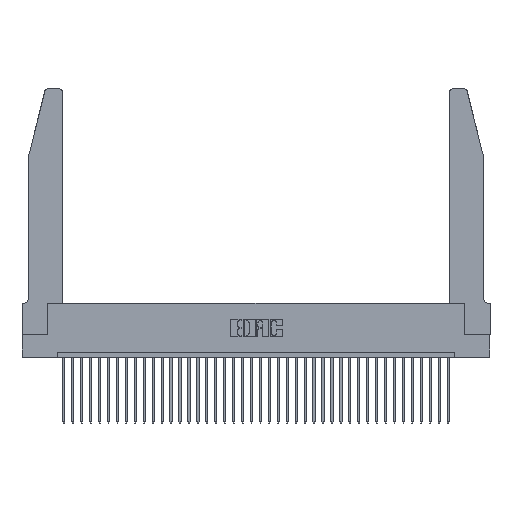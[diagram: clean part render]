
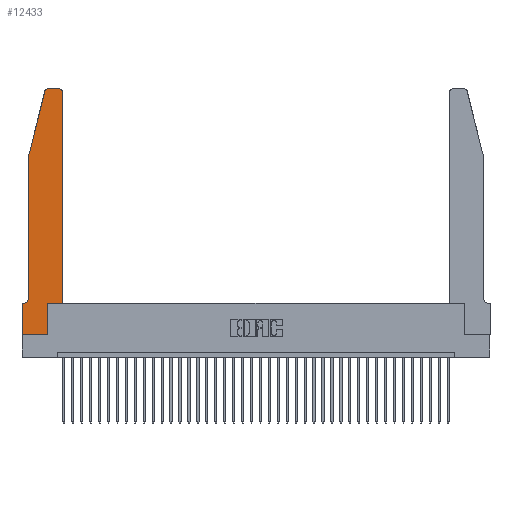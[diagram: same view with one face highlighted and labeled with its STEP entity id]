
A CAD part, top view. The second image highlights one B-rep face of the part: STEP entity #12433.
In plain terms, the highlighted planar face has unit normal (0, 0, 1).
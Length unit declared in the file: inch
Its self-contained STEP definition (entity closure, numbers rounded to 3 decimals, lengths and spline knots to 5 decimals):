
#26 = DIRECTION ( 'NONE',  ( -1., 0., 0. ) ) ;
#142 = DIRECTION ( 'NONE',  ( 0., 0., -1. ) ) ;
#622 = VERTEX_POINT ( 'NONE', #20012 ) ;
#1090 = CARTESIAN_POINT ( 'NONE',  ( 0.0755, 2., 0.37 ) ) ;
#2080 = EDGE_CURVE ( 'NONE', #25891, #23656, #34438, .T. ) ;
#2260 = CARTESIAN_POINT ( 'NONE',  ( 0.2865, 0.35, 0.37 ) ) ;
#3184 = ORIENTED_EDGE ( 'NONE', *, *, #5384, .T. ) ;
#3416 = VECTOR ( 'NONE', #31844, 39.37008 ) ;
#3446 = CARTESIAN_POINT ( 'NONE',  ( 0.4505, 2.72, 0.37 ) ) ;
#4374 = DIRECTION ( 'NONE',  ( 1., 0., 0. ) ) ;
#4702 = PLANE ( 'NONE',  #23932 ) ;
#4921 = VECTOR ( 'NONE', #36363, 39.37008 ) ;
#5002 = LINE ( 'NONE', #12456, #34992 ) ;
#5061 = ORIENTED_EDGE ( 'NONE', *, *, #16618, .T. ) ;
#5384 = EDGE_CURVE ( 'NONE', #24776, #35681, #33946, .T. ) ;
#5389 = VERTEX_POINT ( 'NONE', #29355 ) ;
#5837 = EDGE_CURVE ( 'NONE', #5389, #24776, #26176, .T. ) ;
#6209 = AXIS2_PLACEMENT_3D ( 'NONE', #10601, #16093, #4374 ) ;
#7248 = ORIENTED_EDGE ( 'NONE', *, *, #21227, .T. ) ;
#7262 = VECTOR ( 'NONE', #21818, 39.37008 ) ;
#7862 = CARTESIAN_POINT ( 'NONE',  ( 0.0055, 0.42, 0.37 ) ) ;
#8034 = CARTESIAN_POINT ( 'NONE',  ( 0., 0., 0.37 ) ) ;
#8630 = CIRCLE ( 'NONE', #18538, 0.07 ) ;
#8781 = CARTESIAN_POINT ( 'NONE',  ( 0.0055, 0.35, 0.37 ) ) ;
#8785 = EDGE_LOOP ( 'NONE', ( #16765, #20281, #16480, #3184, #7248, #9335, #5061, #36417, #18719, #33407, #26424, #9458 ) ) ;
#9014 = DIRECTION ( 'NONE',  ( 0., -1., 0. ) ) ;
#9170 = EDGE_CURVE ( 'NONE', #14388, #25891, #5002, .T. ) ;
#9207 = LINE ( 'NONE', #15293, #27850 ) ;
#9335 = ORIENTED_EDGE ( 'NONE', *, *, #14535, .T. ) ;
#9458 = ORIENTED_EDGE ( 'NONE', *, *, #36519, .T. ) ;
#10260 = CARTESIAN_POINT ( 'NONE',  ( 0., 0., 0.37 ) ) ;
#10601 = CARTESIAN_POINT ( 'NONE',  ( 0.284, 2.72, 0.37 ) ) ;
#10736 = CARTESIAN_POINT ( 'NONE',  ( 0.4505, 0.35, 0.37 ) ) ;
#11313 = EDGE_CURVE ( 'NONE', #13683, #11473, #19161, .T. ) ;
#11473 = VERTEX_POINT ( 'NONE', #37413 ) ;
#11820 = DIRECTION ( 'NONE',  ( 0., 0., 1. ) ) ;
#12433 = ADVANCED_FACE ( 'NONE', ( #17025 ), #4702, .T. ) ;
#12456 = CARTESIAN_POINT ( 'NONE',  ( 0.4505, 0.35, 0.37 ) ) ;
#12545 = EDGE_CURVE ( 'NONE', #25888, #22016, #34281, .T. ) ;
#13468 = DIRECTION ( 'NONE',  ( 0., 0., 1. ) ) ;
#13683 = VERTEX_POINT ( 'NONE', #8034 ) ;
#13939 = CIRCLE ( 'NONE', #15026, 0.03 ) ;
#14279 = VERTEX_POINT ( 'NONE', #8781 ) ;
#14388 = VERTEX_POINT ( 'NONE', #2260 ) ;
#14535 = EDGE_CURVE ( 'NONE', #14279, #622, #29141, .T. ) ;
#15026 = AXIS2_PLACEMENT_3D ( 'NONE', #23036, #11820, #17715 ) ;
#15293 = CARTESIAN_POINT ( 'NONE',  ( 0.2865, 0.35, 0.37 ) ) ;
#15770 = VECTOR ( 'NONE', #9014, 39.37008 ) ;
#16093 = DIRECTION ( 'NONE',  ( 0., 0., 1. ) ) ;
#16480 = ORIENTED_EDGE ( 'NONE', *, *, #5837, .T. ) ;
#16618 = EDGE_CURVE ( 'NONE', #622, #13683, #26628, .T. ) ;
#16765 = ORIENTED_EDGE ( 'NONE', *, *, #12545, .T. ) ;
#17025 = FACE_OUTER_BOUND ( 'NONE', #8785, .T. ) ;
#17715 = DIRECTION ( 'NONE',  ( 1., 0., 0. ) ) ;
#18538 = AXIS2_PLACEMENT_3D ( 'NONE', #7862, #142, #26 ) ;
#18719 = ORIENTED_EDGE ( 'NONE', *, *, #26531, .T. ) ;
#18744 = CARTESIAN_POINT ( 'NONE',  ( 0.4505, 0.35, 0.37 ) ) ;
#19161 = LINE ( 'NONE', #25100, #7262 ) ;
#19761 = CARTESIAN_POINT ( 'NONE',  ( 0.4205, 2.75, 0.37 ) ) ;
#20012 = CARTESIAN_POINT ( 'NONE',  ( 0., 0.35, 0.37 ) ) ;
#20281 = ORIENTED_EDGE ( 'NONE', *, *, #36299, .T. ) ;
#20335 = CARTESIAN_POINT ( 'NONE',  ( 0.0755, 0.35, 0.37 ) ) ;
#21227 = EDGE_CURVE ( 'NONE', #35681, #14279, #8630, .T. ) ;
#21818 = DIRECTION ( 'NONE',  ( 1., 0., 0. ) ) ;
#21905 = DIRECTION ( 'NONE',  ( 1., 0., 0. ) ) ;
#22016 = VERTEX_POINT ( 'NONE', #23420 ) ;
#23036 = CARTESIAN_POINT ( 'NONE',  ( 0.4205, 2.72, 0.37 ) ) ;
#23420 = CARTESIAN_POINT ( 'NONE',  ( 0.284, 2.75, 0.37 ) ) ;
#23656 = VERTEX_POINT ( 'NONE', #3446 ) ;
#23932 = AXIS2_PLACEMENT_3D ( 'NONE', #30872, #13468, #21905 ) ;
#24088 = CIRCLE ( 'NONE', #6209, 0.03 ) ;
#24591 = VECTOR ( 'NONE', #34892, 39.37008 ) ;
#24765 = VECTOR ( 'NONE', #37328, 39.37008 ) ;
#24776 = VERTEX_POINT ( 'NONE', #1090 ) ;
#25100 = CARTESIAN_POINT ( 'NONE',  ( 0., 0., 0.37 ) ) ;
#25888 = VERTEX_POINT ( 'NONE', #19761 ) ;
#25891 = VERTEX_POINT ( 'NONE', #10736 ) ;
#26176 = LINE ( 'NONE', #32086, #3416 ) ;
#26207 = VECTOR ( 'NONE', #30218, 39.37008 ) ;
#26424 = ORIENTED_EDGE ( 'NONE', *, *, #2080, .T. ) ;
#26531 = EDGE_CURVE ( 'NONE', #11473, #14388, #9207, .T. ) ;
#26628 = LINE ( 'NONE', #10260, #26207 ) ;
#27850 = VECTOR ( 'NONE', #35589, 39.37008 ) ;
#28968 = DIRECTION ( 'NONE',  ( 1., 0., 0. ) ) ;
#29141 = LINE ( 'NONE', #20335, #24591 ) ;
#29355 = CARTESIAN_POINT ( 'NONE',  ( 0.25487, 2.72718, 0.37 ) ) ;
#30218 = DIRECTION ( 'NONE',  ( 0., -1., 0. ) ) ;
#30872 = CARTESIAN_POINT ( 'NONE',  ( 0., 0.35, 0.37 ) ) ;
#31112 = CARTESIAN_POINT ( 'NONE',  ( 0.2605, 2.75, 0.37 ) ) ;
#31844 = DIRECTION ( 'NONE',  ( -0.239, -0.971, 0. ) ) ;
#32086 = CARTESIAN_POINT ( 'NONE',  ( 0.0755, 2., 0.37 ) ) ;
#32485 = CARTESIAN_POINT ( 'NONE',  ( 0.0755, 2., 0.37 ) ) ;
#33407 = ORIENTED_EDGE ( 'NONE', *, *, #9170, .T. ) ;
#33946 = LINE ( 'NONE', #32485, #15770 ) ;
#34281 = LINE ( 'NONE', #31112, #24765 ) ;
#34438 = LINE ( 'NONE', #18744, #4921 ) ;
#34892 = DIRECTION ( 'NONE',  ( -1., 0., 0. ) ) ;
#34992 = VECTOR ( 'NONE', #28968, 39.37008 ) ;
#35589 = DIRECTION ( 'NONE',  ( 0., 1., 0. ) ) ;
#35681 = VERTEX_POINT ( 'NONE', #36172 ) ;
#36172 = CARTESIAN_POINT ( 'NONE',  ( 0.0755, 0.42, 0.37 ) ) ;
#36299 = EDGE_CURVE ( 'NONE', #22016, #5389, #24088, .T. ) ;
#36363 = DIRECTION ( 'NONE',  ( 0., 1., 0. ) ) ;
#36417 = ORIENTED_EDGE ( 'NONE', *, *, #11313, .T. ) ;
#36519 = EDGE_CURVE ( 'NONE', #23656, #25888, #13939, .T. ) ;
#37328 = DIRECTION ( 'NONE',  ( -1., 0., 0. ) ) ;
#37413 = CARTESIAN_POINT ( 'NONE',  ( 0.2865, 0., 0.37 ) ) ;
